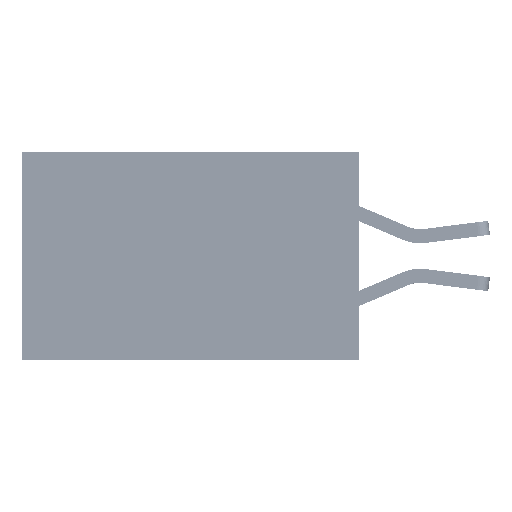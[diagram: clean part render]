
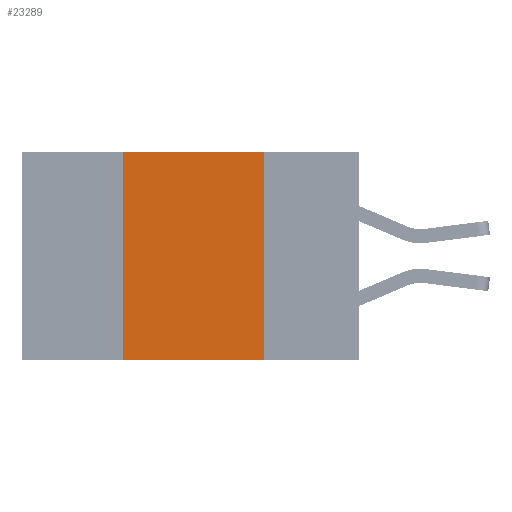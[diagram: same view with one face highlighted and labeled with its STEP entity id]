
A CAD part, left-side view. The second image highlights one B-rep face of the part: STEP entity #23289.
In plain terms, the highlighted planar face has unit normal (-1, 0, 0).
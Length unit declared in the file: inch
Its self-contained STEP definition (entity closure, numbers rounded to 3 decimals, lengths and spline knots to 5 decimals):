
#473 = CARTESIAN_POINT ( 'NONE',  ( 0., 0.42, 0. ) ) ;
#732 = CARTESIAN_POINT ( 'NONE',  ( 0., 0.6, 0. ) ) ;
#1847 = VERTEX_POINT ( 'NONE', #39065 ) ;
#1937 = PLANE ( 'NONE',  #19881 ) ;
#3478 = DIRECTION ( 'NONE',  ( 0., 0., -1. ) ) ;
#4846 = FACE_OUTER_BOUND ( 'NONE', #40952, .T. ) ;
#8802 = ORIENTED_EDGE ( 'NONE', *, *, #22867, .F. ) ;
#10324 = VECTOR ( 'NONE', #19066, 39.37008 ) ;
#13513 = EDGE_CURVE ( 'NONE', #1847, #43107, #18499, .T. ) ;
#13531 = VERTEX_POINT ( 'NONE', #38905 ) ;
#15581 = CARTESIAN_POINT ( 'NONE',  ( 0., 0.6, -0.37 ) ) ;
#16047 = DIRECTION ( 'NONE',  ( 1., 0., 0. ) ) ;
#17426 = VECTOR ( 'NONE', #21396, 39.37008 ) ;
#18160 = VECTOR ( 'NONE', #25160, 39.37008 ) ;
#18499 = LINE ( 'NONE', #473, #17426 ) ;
#19066 = DIRECTION ( 'NONE',  ( 0., -1., 0. ) ) ;
#19200 = ORIENTED_EDGE ( 'NONE', *, *, #13513, .F. ) ;
#19881 = AXIS2_PLACEMENT_3D ( 'NONE', #36897, #16047, #40362 ) ;
#19903 = EDGE_CURVE ( 'NONE', #43107, #13531, #36706, .T. ) ;
#21396 = DIRECTION ( 'NONE',  ( 0., 0., 1. ) ) ;
#22511 = ORIENTED_EDGE ( 'NONE', *, *, #23215, .T. ) ;
#22675 = VERTEX_POINT ( 'NONE', #25868 ) ;
#22867 = EDGE_CURVE ( 'NONE', #13531, #22675, #23483, .T. ) ;
#23215 = EDGE_CURVE ( 'NONE', #1847, #22675, #36011, .T. ) ;
#23289 = ADVANCED_FACE ( 'NONE', ( #4846 ), #1937, .F. ) ;
#23483 = LINE ( 'NONE', #38275, #40868 ) ;
#25160 = DIRECTION ( 'NONE',  ( 0., -1., 0. ) ) ;
#25868 = CARTESIAN_POINT ( 'NONE',  ( 0., 0.17, -0.37 ) ) ;
#36011 = LINE ( 'NONE', #15581, #10324 ) ;
#36667 = ORIENTED_EDGE ( 'NONE', *, *, #19903, .F. ) ;
#36706 = LINE ( 'NONE', #732, #18160 ) ;
#36777 = CARTESIAN_POINT ( 'NONE',  ( 0., 0.42, 0. ) ) ;
#36897 = CARTESIAN_POINT ( 'NONE',  ( 0., 0.6, 0. ) ) ;
#38275 = CARTESIAN_POINT ( 'NONE',  ( 0., 0.17, 0. ) ) ;
#38905 = CARTESIAN_POINT ( 'NONE',  ( 0., 0.17, 0. ) ) ;
#39065 = CARTESIAN_POINT ( 'NONE',  ( 0., 0.42, -0.37 ) ) ;
#40362 = DIRECTION ( 'NONE',  ( 0., 0., -1. ) ) ;
#40868 = VECTOR ( 'NONE', #3478, 39.37008 ) ;
#40952 = EDGE_LOOP ( 'NONE', ( #8802, #36667, #19200, #22511 ) ) ;
#43107 = VERTEX_POINT ( 'NONE', #36777 ) ;
